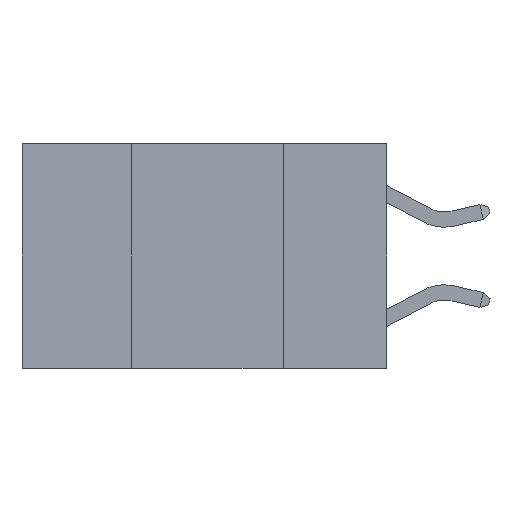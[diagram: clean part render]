
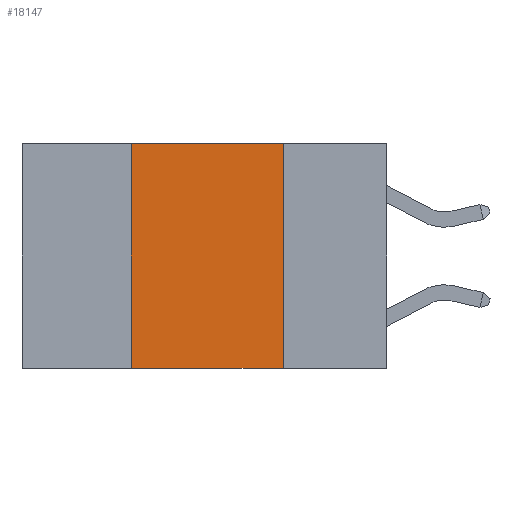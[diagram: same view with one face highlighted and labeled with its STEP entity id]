
A CAD part, left-side view. The second image highlights one B-rep face of the part: STEP entity #18147.
In plain terms, the highlighted planar face has unit normal (-1, 0, 0).
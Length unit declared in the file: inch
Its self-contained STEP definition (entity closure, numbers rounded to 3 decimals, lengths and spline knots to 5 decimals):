
#895 = VECTOR ( 'NONE', #22469, 39.37008 ) ;
#1046 = VECTOR ( 'NONE', #4890, 39.37008 ) ;
#2956 = ORIENTED_EDGE ( 'NONE', *, *, #24629, .F. ) ;
#4890 = DIRECTION ( 'NONE',  ( 0., 0., 1. ) ) ;
#5055 = CARTESIAN_POINT ( 'NONE',  ( 0., 0.6, 0. ) ) ;
#6568 = CARTESIAN_POINT ( 'NONE',  ( 0., 0.42, 0. ) ) ;
#6997 = DIRECTION ( 'NONE',  ( 0., 0., -1. ) ) ;
#8198 = VERTEX_POINT ( 'NONE', #6568 ) ;
#8280 = EDGE_CURVE ( 'NONE', #18931, #14362, #20442, .T. ) ;
#8879 = CARTESIAN_POINT ( 'NONE',  ( 0., 0.17, 0. ) ) ;
#9055 = FACE_OUTER_BOUND ( 'NONE', #20865, .T. ) ;
#10376 = DIRECTION ( 'NONE',  ( 0., -1., 0. ) ) ;
#10780 = LINE ( 'NONE', #18440, #1046 ) ;
#11218 = CARTESIAN_POINT ( 'NONE',  ( 0., 0.17, 0. ) ) ;
#12704 = PLANE ( 'NONE',  #24721 ) ;
#12918 = CARTESIAN_POINT ( 'NONE',  ( 0., 0.17, -0.37 ) ) ;
#13232 = ORIENTED_EDGE ( 'NONE', *, *, #8280, .T. ) ;
#14362 = VERTEX_POINT ( 'NONE', #12918 ) ;
#14731 = CARTESIAN_POINT ( 'NONE',  ( 0., 0.42, -0.37 ) ) ;
#15017 = EDGE_CURVE ( 'NONE', #15158, #14362, #16367, .T. ) ;
#15158 = VERTEX_POINT ( 'NONE', #11218 ) ;
#15507 = ORIENTED_EDGE ( 'NONE', *, *, #15541, .F. ) ;
#15541 = EDGE_CURVE ( 'NONE', #8198, #15158, #22198, .T. ) ;
#16367 = LINE ( 'NONE', #8879, #895 ) ;
#17899 = ORIENTED_EDGE ( 'NONE', *, *, #15017, .F. ) ;
#18147 = ADVANCED_FACE ( 'NONE', ( #9055 ), #12704, .F. ) ;
#18406 = DIRECTION ( 'NONE',  ( 0., -1., 0. ) ) ;
#18440 = CARTESIAN_POINT ( 'NONE',  ( 0., 0.42, 0. ) ) ;
#18600 = DIRECTION ( 'NONE',  ( 1., 0., 0. ) ) ;
#18931 = VERTEX_POINT ( 'NONE', #14731 ) ;
#19112 = VECTOR ( 'NONE', #10376, 39.37008 ) ;
#19836 = VECTOR ( 'NONE', #18406, 39.37008 ) ;
#20442 = LINE ( 'NONE', #22270, #19836 ) ;
#20865 = EDGE_LOOP ( 'NONE', ( #17899, #15507, #2956, #13232 ) ) ;
#22198 = LINE ( 'NONE', #23983, #19112 ) ;
#22270 = CARTESIAN_POINT ( 'NONE',  ( 0., 0.6, -0.37 ) ) ;
#22469 = DIRECTION ( 'NONE',  ( 0., 0., -1. ) ) ;
#23983 = CARTESIAN_POINT ( 'NONE',  ( 0., 0.6, 0. ) ) ;
#24629 = EDGE_CURVE ( 'NONE', #18931, #8198, #10780, .T. ) ;
#24721 = AXIS2_PLACEMENT_3D ( 'NONE', #5055, #18600, #6997 ) ;
